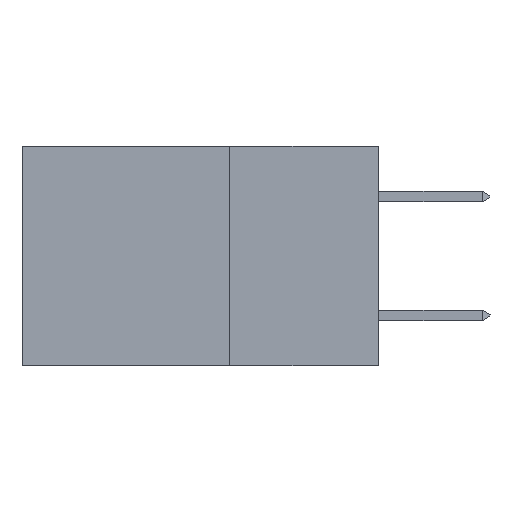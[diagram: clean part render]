
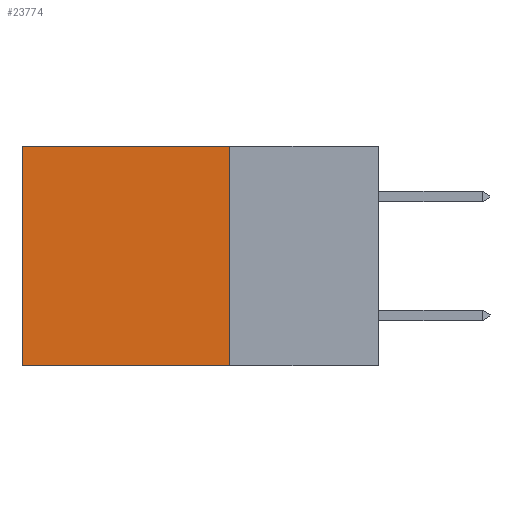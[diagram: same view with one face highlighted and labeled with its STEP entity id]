
A CAD part, left-side view. The second image highlights one B-rep face of the part: STEP entity #23774.
In plain terms, the highlighted planar face has unit normal (-1, 0, 0).
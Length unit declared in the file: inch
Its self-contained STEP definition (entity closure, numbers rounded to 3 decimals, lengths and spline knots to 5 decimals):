
#1317 = EDGE_CURVE ( 'NONE', #13426, #10075, #13365, .T. ) ;
#2577 = VERTEX_POINT ( 'NONE', #7213 ) ;
#2767 = VECTOR ( 'NONE', #5708, 39.37008 ) ;
#3485 = EDGE_CURVE ( 'NONE', #10075, #21528, #8332, .T. ) ;
#3678 = CARTESIAN_POINT ( 'NONE',  ( 0.2615, 0.6, -0.37 ) ) ;
#5075 = CARTESIAN_POINT ( 'NONE',  ( 0.2615, 0.25, -0.37 ) ) ;
#5708 = DIRECTION ( 'NONE',  ( 0., 0., -1. ) ) ;
#6663 = ORIENTED_EDGE ( 'NONE', *, *, #3485, .F. ) ;
#7213 = CARTESIAN_POINT ( 'NONE',  ( 0.2615, 0.6, 0. ) ) ;
#7605 = EDGE_LOOP ( 'NONE', ( #22252, #6663, #12952, #23575 ) ) ;
#7872 = DIRECTION ( 'NONE',  ( 0., 0., -1. ) ) ;
#8125 = VECTOR ( 'NONE', #7872, 39.37008 ) ;
#8332 = LINE ( 'NONE', #8478, #12349 ) ;
#8478 = CARTESIAN_POINT ( 'NONE',  ( 0.2615, 0.25, -0.37 ) ) ;
#9357 = EDGE_CURVE ( 'NONE', #13426, #2577, #24262, .T. ) ;
#10075 = VERTEX_POINT ( 'NONE', #17394 ) ;
#11661 = CARTESIAN_POINT ( 'NONE',  ( 0.2615, 0.25, 0. ) ) ;
#12349 = VECTOR ( 'NONE', #23871, 39.37008 ) ;
#12733 = FACE_OUTER_BOUND ( 'NONE', #7605, .T. ) ;
#12952 = ORIENTED_EDGE ( 'NONE', *, *, #1317, .F. ) ;
#13080 = DIRECTION ( 'NONE',  ( 0., 0., -1. ) ) ;
#13365 = LINE ( 'NONE', #17163, #8125 ) ;
#13380 = LINE ( 'NONE', #3678, #2767 ) ;
#13426 = VERTEX_POINT ( 'NONE', #14637 ) ;
#14637 = CARTESIAN_POINT ( 'NONE',  ( 0.2615, 0.25, 0. ) ) ;
#16010 = AXIS2_PLACEMENT_3D ( 'NONE', #5075, #24456, #13080 ) ;
#16022 = EDGE_CURVE ( 'NONE', #2577, #21528, #13380, .T. ) ;
#17163 = CARTESIAN_POINT ( 'NONE',  ( 0.2615, 0.25, -0.37 ) ) ;
#17394 = CARTESIAN_POINT ( 'NONE',  ( 0.2615, 0.25, -0.37 ) ) ;
#19226 = VECTOR ( 'NONE', #23082, 39.37008 ) ;
#21528 = VERTEX_POINT ( 'NONE', #22070 ) ;
#22070 = CARTESIAN_POINT ( 'NONE',  ( 0.2615, 0.6, -0.37 ) ) ;
#22252 = ORIENTED_EDGE ( 'NONE', *, *, #16022, .T. ) ;
#22565 = PLANE ( 'NONE',  #16010 ) ;
#23082 = DIRECTION ( 'NONE',  ( 0., 1., 0. ) ) ;
#23575 = ORIENTED_EDGE ( 'NONE', *, *, #9357, .T. ) ;
#23774 = ADVANCED_FACE ( 'NONE', ( #12733 ), #22565, .F. ) ;
#23871 = DIRECTION ( 'NONE',  ( 0., 1., 0. ) ) ;
#24262 = LINE ( 'NONE', #11661, #19226 ) ;
#24456 = DIRECTION ( 'NONE',  ( 1., 0., 0. ) ) ;
